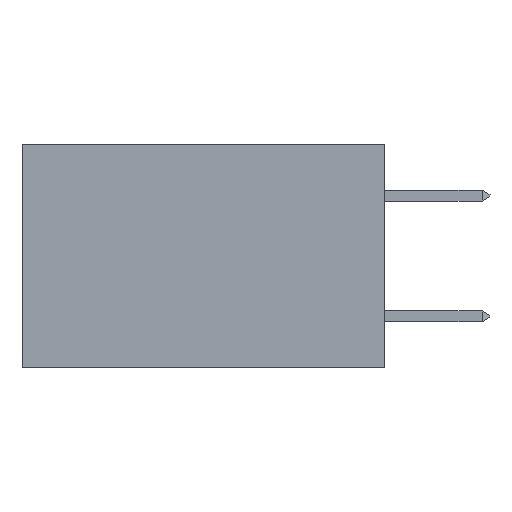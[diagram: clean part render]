
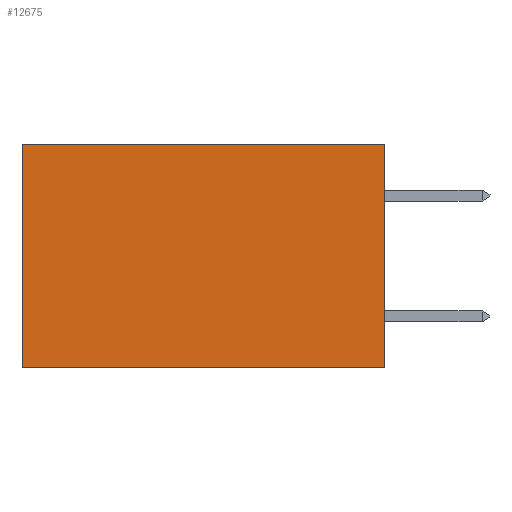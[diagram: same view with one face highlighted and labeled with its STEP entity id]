
A CAD part, left-side view. The second image highlights one B-rep face of the part: STEP entity #12675.
In plain terms, the highlighted planar face has unit normal (-1, 0, 0).
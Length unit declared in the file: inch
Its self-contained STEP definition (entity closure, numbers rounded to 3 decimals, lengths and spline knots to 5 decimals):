
#664 = DIRECTION ( 'NONE',  ( 0., 1., 0. ) ) ;
#815 = DIRECTION ( 'NONE',  ( 0., 1., 0. ) ) ;
#2927 = ORIENTED_EDGE ( 'NONE', *, *, #10154, .T. ) ;
#4860 = CARTESIAN_POINT ( 'NONE',  ( 0.2875, 0., 0. ) ) ;
#5974 = ORIENTED_EDGE ( 'NONE', *, *, #10074, .T. ) ;
#6423 = VECTOR ( 'NONE', #664, 39.37008 ) ;
#6901 = PLANE ( 'NONE',  #13036 ) ;
#7671 = VERTEX_POINT ( 'NONE', #18264 ) ;
#8769 = DIRECTION ( 'NONE',  ( 1., 0., 0. ) ) ;
#8934 = DIRECTION ( 'NONE',  ( 0., 0., -1. ) ) ;
#9554 = VERTEX_POINT ( 'NONE', #13136 ) ;
#10074 = EDGE_CURVE ( 'NONE', #23781, #9554, #18081, .T. ) ;
#10154 = EDGE_CURVE ( 'NONE', #9554, #18764, #24760, .T. ) ;
#10729 = DIRECTION ( 'NONE',  ( 0., 0., -1. ) ) ;
#12675 = ADVANCED_FACE ( 'NONE', ( #20637 ), #6901, .F. ) ;
#12950 = VECTOR ( 'NONE', #815, 39.37008 ) ;
#13036 = AXIS2_PLACEMENT_3D ( 'NONE', #24389, #8769, #8934 ) ;
#13136 = CARTESIAN_POINT ( 'NONE',  ( 0.2875, 0.6, 0. ) ) ;
#13228 = VECTOR ( 'NONE', #17464, 39.37008 ) ;
#13353 = LINE ( 'NONE', #14044, #6423 ) ;
#13577 = CARTESIAN_POINT ( 'NONE',  ( 0.2875, 0., 0. ) ) ;
#14044 = CARTESIAN_POINT ( 'NONE',  ( 0.2875, 0., -0.37 ) ) ;
#14338 = ORIENTED_EDGE ( 'NONE', *, *, #18252, .F. ) ;
#15298 = ORIENTED_EDGE ( 'NONE', *, *, #21752, .F. ) ;
#17464 = DIRECTION ( 'NONE',  ( 0., 0., -1. ) ) ;
#18081 = LINE ( 'NONE', #4860, #12950 ) ;
#18252 = EDGE_CURVE ( 'NONE', #23781, #7671, #21040, .T. ) ;
#18264 = CARTESIAN_POINT ( 'NONE',  ( 0.2875, 0., -0.37 ) ) ;
#18764 = VERTEX_POINT ( 'NONE', #20808 ) ;
#20528 = EDGE_LOOP ( 'NONE', ( #2927, #15298, #14338, #5974 ) ) ;
#20637 = FACE_OUTER_BOUND ( 'NONE', #20528, .T. ) ;
#20808 = CARTESIAN_POINT ( 'NONE',  ( 0.2875, 0.6, -0.37 ) ) ;
#21040 = LINE ( 'NONE', #13577, #13228 ) ;
#21752 = EDGE_CURVE ( 'NONE', #7671, #18764, #13353, .T. ) ;
#21796 = CARTESIAN_POINT ( 'NONE',  ( 0.2875, 0., 0. ) ) ;
#22275 = CARTESIAN_POINT ( 'NONE',  ( 0.2875, 0.6, 0. ) ) ;
#22297 = VECTOR ( 'NONE', #10729, 39.37008 ) ;
#23781 = VERTEX_POINT ( 'NONE', #21796 ) ;
#24389 = CARTESIAN_POINT ( 'NONE',  ( 0.2875, 0., 0. ) ) ;
#24760 = LINE ( 'NONE', #22275, #22297 ) ;
